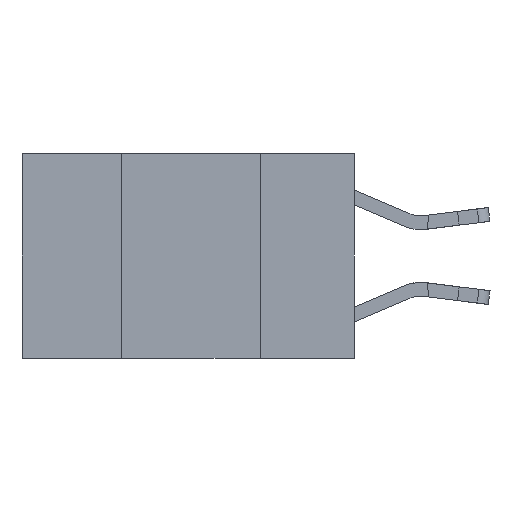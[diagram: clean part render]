
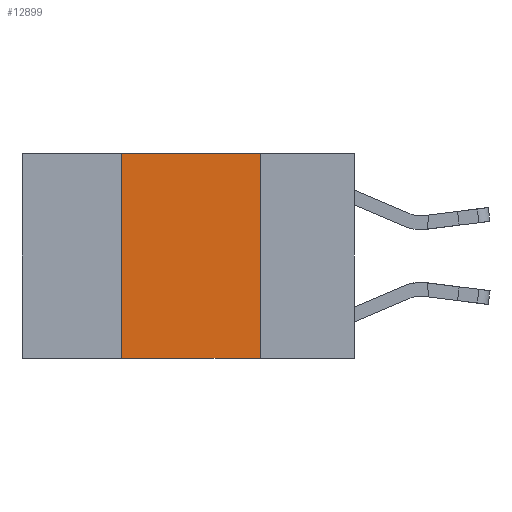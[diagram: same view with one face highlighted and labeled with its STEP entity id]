
A CAD part, left-side view. The second image highlights one B-rep face of the part: STEP entity #12899.
In plain terms, the highlighted planar face has unit normal (-1, 0, 0).
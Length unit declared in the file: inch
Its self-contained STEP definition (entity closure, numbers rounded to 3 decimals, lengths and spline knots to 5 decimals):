
#69 = DIRECTION ( 'NONE',  ( 0., -1., 0. ) ) ;
#182 = EDGE_CURVE ( 'NONE', #3125, #11935, #889, .T. ) ;
#889 = LINE ( 'NONE', #17923, #7781 ) ;
#1180 = LINE ( 'NONE', #14188, #12359 ) ;
#1199 = EDGE_CURVE ( 'NONE', #7447, #5369, #8120, .T. ) ;
#1563 = EDGE_LOOP ( 'NONE', ( #4086, #16231, #15933, #13942 ) ) ;
#1762 = EDGE_CURVE ( 'NONE', #3125, #5369, #15847, .T. ) ;
#2506 = EDGE_CURVE ( 'NONE', #11935, #7447, #1180, .T. ) ;
#3125 = VERTEX_POINT ( 'NONE', #10468 ) ;
#3409 = DIRECTION ( 'NONE',  ( 0., -1., 0. ) ) ;
#3507 = VECTOR ( 'NONE', #18061, 39.37008 ) ;
#4086 = ORIENTED_EDGE ( 'NONE', *, *, #1199, .F. ) ;
#4722 = CARTESIAN_POINT ( 'NONE',  ( 0., 0.17, -0.37 ) ) ;
#5369 = VERTEX_POINT ( 'NONE', #4722 ) ;
#6711 = FACE_OUTER_BOUND ( 'NONE', #1563, .T. ) ;
#7000 = VECTOR ( 'NONE', #3409, 39.37008 ) ;
#7447 = VERTEX_POINT ( 'NONE', #11404 ) ;
#7781 = VECTOR ( 'NONE', #15285, 39.37008 ) ;
#8089 = AXIS2_PLACEMENT_3D ( 'NONE', #14023, #16814, #12592 ) ;
#8120 = LINE ( 'NONE', #8208, #3507 ) ;
#8208 = CARTESIAN_POINT ( 'NONE',  ( 0., 0.17, 0. ) ) ;
#10468 = CARTESIAN_POINT ( 'NONE',  ( 0., 0.42, -0.37 ) ) ;
#11081 = PLANE ( 'NONE',  #8089 ) ;
#11404 = CARTESIAN_POINT ( 'NONE',  ( 0., 0.17, 0. ) ) ;
#11935 = VERTEX_POINT ( 'NONE', #13996 ) ;
#12359 = VECTOR ( 'NONE', #69, 39.37008 ) ;
#12592 = DIRECTION ( 'NONE',  ( 0., 0., -1. ) ) ;
#12899 = ADVANCED_FACE ( 'NONE', ( #6711 ), #11081, .F. ) ;
#13942 = ORIENTED_EDGE ( 'NONE', *, *, #1762, .T. ) ;
#13996 = CARTESIAN_POINT ( 'NONE',  ( 0., 0.42, 0. ) ) ;
#14023 = CARTESIAN_POINT ( 'NONE',  ( 0., 0.6, 0. ) ) ;
#14188 = CARTESIAN_POINT ( 'NONE',  ( 0., 0.6, 0. ) ) ;
#15285 = DIRECTION ( 'NONE',  ( 0., 0., 1. ) ) ;
#15847 = LINE ( 'NONE', #16218, #7000 ) ;
#15933 = ORIENTED_EDGE ( 'NONE', *, *, #182, .F. ) ;
#16218 = CARTESIAN_POINT ( 'NONE',  ( 0., 0.6, -0.37 ) ) ;
#16231 = ORIENTED_EDGE ( 'NONE', *, *, #2506, .F. ) ;
#16814 = DIRECTION ( 'NONE',  ( 1., 0., 0. ) ) ;
#17923 = CARTESIAN_POINT ( 'NONE',  ( 0., 0.42, 0. ) ) ;
#18061 = DIRECTION ( 'NONE',  ( 0., 0., -1. ) ) ;
